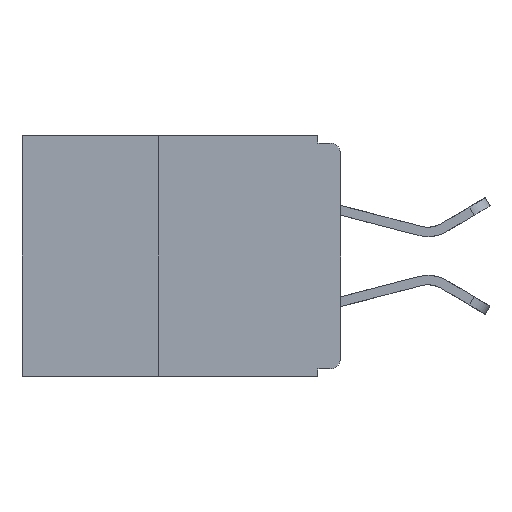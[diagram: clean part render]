
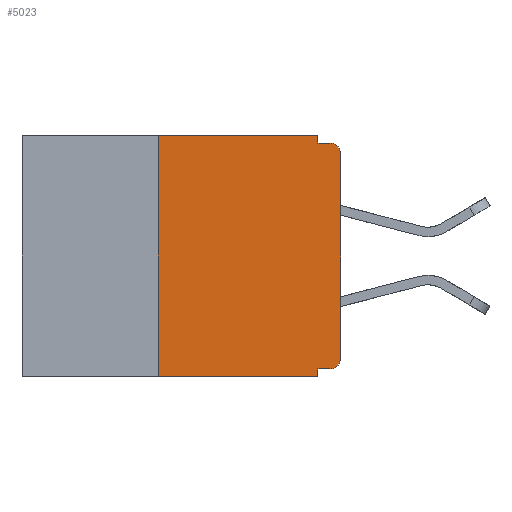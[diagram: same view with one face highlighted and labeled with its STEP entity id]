
A CAD part, left-side view. The second image highlights one B-rep face of the part: STEP entity #5023.
In plain terms, the highlighted planar face has unit normal (-1, 0, 0).
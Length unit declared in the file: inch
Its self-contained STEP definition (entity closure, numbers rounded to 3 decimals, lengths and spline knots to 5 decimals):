
#68 = CARTESIAN_POINT ( 'NONE',  ( 0., 0.25, -0.33 ) ) ;
#87 = PLANE ( 'NONE',  #10760 ) ;
#391 = DIRECTION ( 'NONE',  ( 0., 0., -1. ) ) ;
#415 = ORIENTED_EDGE ( 'NONE', *, *, #8547, .F. ) ;
#581 = LINE ( 'NONE', #9039, #12421 ) ;
#589 = CARTESIAN_POINT ( 'NONE',  ( 0., 0.437, -0.33 ) ) ;
#691 = LINE ( 'NONE', #13723, #3759 ) ;
#792 = ORIENTED_EDGE ( 'NONE', *, *, #5492, .F. ) ;
#922 = DIRECTION ( 'NONE',  ( 0., 0., -1. ) ) ;
#1226 = DIRECTION ( 'NONE',  ( 1., 0., 0. ) ) ;
#1610 = AXIS2_PLACEMENT_3D ( 'NONE', #14067, #7262, #391 ) ;
#1717 = VERTEX_POINT ( 'NONE', #8402 ) ;
#2058 = CARTESIAN_POINT ( 'NONE',  ( 0., 0., 0. ) ) ;
#2356 = VECTOR ( 'NONE', #922, 39.37008 ) ;
#2382 = CARTESIAN_POINT ( 'NONE',  ( 0., 0.031, -0.32 ) ) ;
#2578 = LINE ( 'NONE', #5548, #11734 ) ;
#2729 = VERTEX_POINT ( 'NONE', #4987 ) ;
#2912 = VERTEX_POINT ( 'NONE', #4226 ) ;
#3596 = CARTESIAN_POINT ( 'NONE',  ( 0., 0.031, -0.01 ) ) ;
#3660 = EDGE_CURVE ( 'NONE', #3812, #5321, #2578, .T. ) ;
#3759 = VECTOR ( 'NONE', #11514, 39.37008 ) ;
#3812 = VERTEX_POINT ( 'NONE', #3596 ) ;
#4048 = ORIENTED_EDGE ( 'NONE', *, *, #11753, .T. ) ;
#4053 = CARTESIAN_POINT ( 'NONE',  ( 0., 0.015, -0.01 ) ) ;
#4226 = CARTESIAN_POINT ( 'NONE',  ( 0., 0.25, 0. ) ) ;
#4844 = ORIENTED_EDGE ( 'NONE', *, *, #8659, .T. ) ;
#4912 = VECTOR ( 'NONE', #5892, 39.37008 ) ;
#4987 = CARTESIAN_POINT ( 'NONE',  ( 0., 0.031, -0.33 ) ) ;
#5023 = ADVANCED_FACE ( 'NONE', ( #5438 ), #87, .F. ) ;
#5321 = VERTEX_POINT ( 'NONE', #4053 ) ;
#5438 = FACE_OUTER_BOUND ( 'NONE', #6311, .T. ) ;
#5492 = EDGE_CURVE ( 'NONE', #5636, #2729, #8471, .T. ) ;
#5548 = CARTESIAN_POINT ( 'NONE',  ( 0., 0., -0.01 ) ) ;
#5636 = VERTEX_POINT ( 'NONE', #2382 ) ;
#5642 = VERTEX_POINT ( 'NONE', #68 ) ;
#5892 = DIRECTION ( 'NONE',  ( 0., 1., 0. ) ) ;
#5935 = LINE ( 'NONE', #2058, #14270 ) ;
#6070 = VECTOR ( 'NONE', #7255, 39.37008 ) ;
#6113 = CARTESIAN_POINT ( 'NONE',  ( 0., 0.031, 0. ) ) ;
#6127 = ORIENTED_EDGE ( 'NONE', *, *, #8397, .F. ) ;
#6311 = EDGE_LOOP ( 'NONE', ( #10041, #4844, #8066, #13587, #13780, #6127, #6858, #792, #415, #4048 ) ) ;
#6724 = VERTEX_POINT ( 'NONE', #12282 ) ;
#6799 = CARTESIAN_POINT ( 'NONE',  ( 0., 0.015, -0.305 ) ) ;
#6858 = ORIENTED_EDGE ( 'NONE', *, *, #10629, .T. ) ;
#7255 = DIRECTION ( 'NONE',  ( 0., 0., -1. ) ) ;
#7262 = DIRECTION ( 'NONE',  ( -1., 0., 0. ) ) ;
#7495 = AXIS2_PLACEMENT_3D ( 'NONE', #6799, #14750, #7966 ) ;
#7848 = DIRECTION ( 'NONE',  ( 0., 0., 1. ) ) ;
#7942 = DIRECTION ( 'NONE',  ( 0., 0., 1. ) ) ;
#7966 = DIRECTION ( 'NONE',  ( 0., 0., -1. ) ) ;
#8066 = ORIENTED_EDGE ( 'NONE', *, *, #3660, .F. ) ;
#8127 = CARTESIAN_POINT ( 'NONE',  ( 0., 0.437, 0. ) ) ;
#8251 = VECTOR ( 'NONE', #8685, 39.37008 ) ;
#8394 = CIRCLE ( 'NONE', #7495, 0.015 ) ;
#8397 = EDGE_CURVE ( 'NONE', #5642, #2912, #581, .T. ) ;
#8402 = CARTESIAN_POINT ( 'NONE',  ( 0., 0., -0.305 ) ) ;
#8471 = LINE ( 'NONE', #11286, #2356 ) ;
#8547 = EDGE_CURVE ( 'NONE', #6724, #5636, #13978, .T. ) ;
#8659 = EDGE_CURVE ( 'NONE', #13592, #5321, #9560, .T. ) ;
#8685 = DIRECTION ( 'NONE',  ( 0., -1., 0. ) ) ;
#9039 = CARTESIAN_POINT ( 'NONE',  ( 0., 0.25, -0.33 ) ) ;
#9122 = CARTESIAN_POINT ( 'NONE',  ( 0., 0., -0.025 ) ) ;
#9274 = DIRECTION ( 'NONE',  ( 0., 0., -1. ) ) ;
#9560 = CIRCLE ( 'NONE', #1610, 0.015 ) ;
#9850 = LINE ( 'NONE', #6113, #6070 ) ;
#10041 = ORIENTED_EDGE ( 'NONE', *, *, #10170, .T. ) ;
#10170 = EDGE_CURVE ( 'NONE', #1717, #13592, #5935, .T. ) ;
#10299 = EDGE_CURVE ( 'NONE', #2912, #13718, #691, .T. ) ;
#10629 = EDGE_CURVE ( 'NONE', #5642, #2729, #11309, .T. ) ;
#10760 = AXIS2_PLACEMENT_3D ( 'NONE', #8127, #1226, #9274 ) ;
#11284 = DIRECTION ( 'NONE',  ( 0., -1., 0. ) ) ;
#11286 = CARTESIAN_POINT ( 'NONE',  ( 0., 0.031, -0.33 ) ) ;
#11309 = LINE ( 'NONE', #589, #8251 ) ;
#11424 = CARTESIAN_POINT ( 'NONE',  ( 0., 0.031, 0. ) ) ;
#11514 = DIRECTION ( 'NONE',  ( 0., -1., 0. ) ) ;
#11606 = CARTESIAN_POINT ( 'NONE',  ( 0., 0., -0.32 ) ) ;
#11734 = VECTOR ( 'NONE', #11284, 39.37008 ) ;
#11753 = EDGE_CURVE ( 'NONE', #6724, #1717, #8394, .T. ) ;
#12282 = CARTESIAN_POINT ( 'NONE',  ( 0., 0.015, -0.32 ) ) ;
#12421 = VECTOR ( 'NONE', #7942, 39.37008 ) ;
#13587 = ORIENTED_EDGE ( 'NONE', *, *, #14637, .F. ) ;
#13592 = VERTEX_POINT ( 'NONE', #9122 ) ;
#13718 = VERTEX_POINT ( 'NONE', #11424 ) ;
#13723 = CARTESIAN_POINT ( 'NONE',  ( 0., 0.437, 0. ) ) ;
#13780 = ORIENTED_EDGE ( 'NONE', *, *, #10299, .F. ) ;
#13978 = LINE ( 'NONE', #11606, #4912 ) ;
#14067 = CARTESIAN_POINT ( 'NONE',  ( 0., 0.015, -0.025 ) ) ;
#14270 = VECTOR ( 'NONE', #7848, 39.37008 ) ;
#14637 = EDGE_CURVE ( 'NONE', #13718, #3812, #9850, .T. ) ;
#14750 = DIRECTION ( 'NONE',  ( -1., 0., 0. ) ) ;
